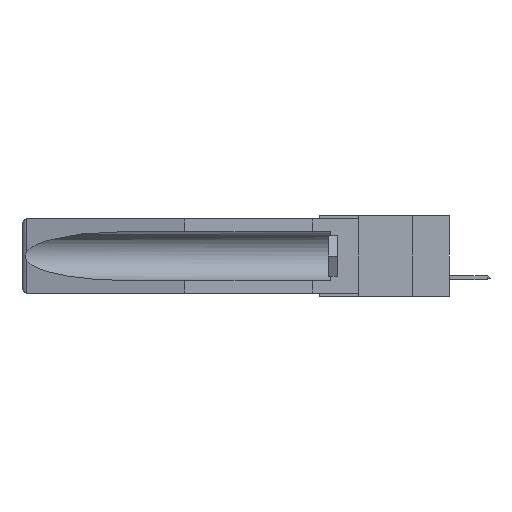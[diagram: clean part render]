
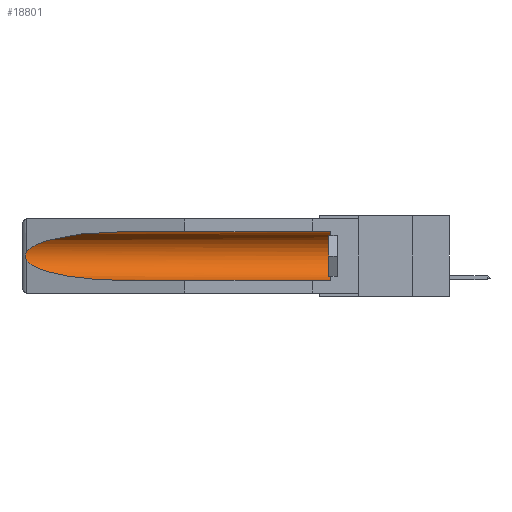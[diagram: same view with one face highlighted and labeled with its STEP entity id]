
A CAD part, left-side view. The second image highlights one B-rep face of the part: STEP entity #18801.
In plain terms, the highlighted cylindrical face has radius 2.857 mm (diameter 5.715 mm), a partial arc.
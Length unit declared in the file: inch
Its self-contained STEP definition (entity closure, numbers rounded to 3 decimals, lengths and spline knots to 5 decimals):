
#703 = VERTEX_POINT ( 'NONE', #5030 ) ;
#1342 = VERTEX_POINT ( 'NONE', #10967 ) ;
#1915 = EDGE_CURVE ( 'NONE', #703, #1342, #19641, .T. ) ;
#2113 = AXIS2_PLACEMENT_3D ( 'NONE', #3444, #9989, #6726 ) ;
#2271 = CIRCLE ( 'NONE', #9163, 0.1125 ) ;
#2732 = DIRECTION ( 'NONE',  ( 0., -1., 0. ) ) ;
#3019 = CARTESIAN_POINT ( 'NONE',  ( 0.25451, 1.48313, -0.09465 ) ) ;
#3235 = CARTESIAN_POINT ( 'NONE',  ( 0.155, 1.07973, -0.059 ) ) ;
#3444 = CARTESIAN_POINT ( 'NONE',  ( 0.155, -0.30754, -0.1715 ) ) ;
#3537 = ORIENTED_EDGE ( 'NONE', *, *, #13903, .F. ) ;
#4358 = LINE ( 'NONE', #16368, #6198 ) ;
#5024 = CARTESIAN_POINT ( 'NONE',  ( 0.26537, 1.52718, -0.14972 ) ) ;
#5030 = CARTESIAN_POINT ( 'NONE',  ( 0.155, 0.126, -0.059 ) ) ;
#6051 = CARTESIAN_POINT ( 'NONE',  ( 0.26654, 1.53092, -0.15636 ) ) ;
#6198 = VECTOR ( 'NONE', #9818, 39.37008 ) ;
#6726 = DIRECTION ( 'NONE',  ( 0., 0., 1. ) ) ;
#7001 = ORIENTED_EDGE ( 'NONE', *, *, #16975, .T. ) ;
#7324 = VERTEX_POINT ( 'NONE', #19945 ) ;
#7453 = CARTESIAN_POINT ( 'NONE',  ( 0.26537, 1.52718, -0.14972 ) ) ;
#7702 = CARTESIAN_POINT ( 'NONE',  ( 0.155, -0.30754, -0.059 ) ) ;
#7738 = CARTESIAN_POINT ( 'NONE',  ( 0.2675, 1.53308, -0.16763 ) ) ;
#7820 = EDGE_LOOP ( 'NONE', ( #7001, #20373, #15381, #3537, #12249, #8042 ) ) ;
#8042 = ORIENTED_EDGE ( 'NONE', *, *, #1915, .T. ) ;
#8125 = VECTOR ( 'NONE', #21120, 39.37008 ) ;
#8310 = CARTESIAN_POINT ( 'NONE',  ( 0.26537, 1.52718, -0.19328 ) ) ;
#9163 = AXIS2_PLACEMENT_3D ( 'NONE', #12665, #2732, #19387 ) ;
#9818 = DIRECTION ( 'NONE',  ( 0., 1., 0. ) ) ;
#9899 = FACE_OUTER_BOUND ( 'NONE', #7820, .T. ) ;
#9965 = B_SPLINE_CURVE_WITH_KNOTS ( 'NONE', 3,
 ( #7453, #12628, #6051, #15957, #7738, #17650, #15746, #10979, #19418, #17429 ),
 .UNSPECIFIED., .F., .F.,
 ( 4, 2, 2, 2, 4 ),
 ( 0., 0.00029, 0.00058, 0.00087, 0.00117 ),
 .UNSPECIFIED. ) ;
#9989 = DIRECTION ( 'NONE',  ( 0., 1., 0. ) ) ;
#10862 = VERTEX_POINT ( 'NONE', #20792 ) ;
#10967 = CARTESIAN_POINT ( 'NONE',  ( 0.155, 1.07973, -0.059 ) ) ;
#10979 = CARTESIAN_POINT ( 'NONE',  ( 0.26655, 1.53094, -0.18657 ) ) ;
#12249 = ORIENTED_EDGE ( 'NONE', *, *, #14209, .T. ) ;
#12628 = CARTESIAN_POINT ( 'NONE',  ( 0.26597, 1.52961, -0.15275 ) ) ;
#12665 = CARTESIAN_POINT ( 'NONE',  ( 0.155, 0.126, -0.1715 ) ) ;
#13320 = CARTESIAN_POINT ( 'NONE',  ( 0.26537, 1.52718, -0.19328 ) ) ;
#13903 = EDGE_CURVE ( 'NONE', #7324, #10862, #4358, .T. ) ;
#14111 = CYLINDRICAL_SURFACE ( 'NONE', #2113, 0.1125 ) ;
#14209 = EDGE_CURVE ( 'NONE', #7324, #703, #2271, .T. ) ;
#15381 = ORIENTED_EDGE ( 'NONE', *, *, #19057, .T. ) ;
#15453 =( BOUNDED_CURVE ( )  B_SPLINE_CURVE ( 3, ( #8310, #16805, #17589, #17446 ),
 .UNSPECIFIED., .F., .T. ) 
 B_SPLINE_CURVE_WITH_KNOTS ( ( 4, 4 ),
 ( 0.1948, 1.5708 ),
 .UNSPECIFIED. ) 
 CURVE ( )  GEOMETRIC_REPRESENTATION_ITEM ( )  RATIONAL_B_SPLINE_CURVE ( ( 1., 0.848, 0.848, 1. ) ) 
 REPRESENTATION_ITEM ( '' )  );
#15746 = CARTESIAN_POINT ( 'NONE',  ( 0.2673, 1.53269, -0.17917 ) ) ;
#15957 = CARTESIAN_POINT ( 'NONE',  ( 0.2673, 1.5327, -0.16383 ) ) ;
#16200 = VERTEX_POINT ( 'NONE', #13320 ) ;
#16368 = CARTESIAN_POINT ( 'NONE',  ( 0.155, -0.30754, -0.284 ) ) ;
#16494 = CARTESIAN_POINT ( 'NONE',  ( 0.26537, 1.52718, -0.14972 ) ) ;
#16805 = CARTESIAN_POINT ( 'NONE',  ( 0.25451, 1.48313, -0.24835 ) ) ;
#16975 = EDGE_CURVE ( 'NONE', #1342, #19453, #17045, .T. ) ;
#17045 =( BOUNDED_CURVE ( )  B_SPLINE_CURVE ( 3, ( #3235, #21423, #3019, #16494 ),
 .UNSPECIFIED., .F., .F. ) 
 B_SPLINE_CURVE_WITH_KNOTS ( ( 4, 4 ),
 ( 4.71239, 6.08839 ),
 .UNSPECIFIED. ) 
 CURVE ( )  GEOMETRIC_REPRESENTATION_ITEM ( )  RATIONAL_B_SPLINE_CURVE ( ( 1., 0.848, 0.848, 1. ) ) 
 REPRESENTATION_ITEM ( '' )  );
#17429 = CARTESIAN_POINT ( 'NONE',  ( 0.26537, 1.52718, -0.19328 ) ) ;
#17446 = CARTESIAN_POINT ( 'NONE',  ( 0.155, 1.07973, -0.284 ) ) ;
#17589 = CARTESIAN_POINT ( 'NONE',  ( 0.21114, 1.30732, -0.284 ) ) ;
#17650 = CARTESIAN_POINT ( 'NONE',  ( 0.2675, 1.53308, -0.17534 ) ) ;
#18801 = ADVANCED_FACE ( 'NONE', ( #9899 ), #14111, .F. ) ;
#19057 = EDGE_CURVE ( 'NONE', #16200, #10862, #15453, .T. ) ;
#19190 = EDGE_CURVE ( 'NONE', #19453, #16200, #9965, .T. ) ;
#19387 = DIRECTION ( 'NONE',  ( 0., 0., 1. ) ) ;
#19418 = CARTESIAN_POINT ( 'NONE',  ( 0.26597, 1.5296, -0.19026 ) ) ;
#19453 = VERTEX_POINT ( 'NONE', #5024 ) ;
#19641 = LINE ( 'NONE', #7702, #8125 ) ;
#19945 = CARTESIAN_POINT ( 'NONE',  ( 0.155, 0.126, -0.284 ) ) ;
#20373 = ORIENTED_EDGE ( 'NONE', *, *, #19190, .T. ) ;
#20792 = CARTESIAN_POINT ( 'NONE',  ( 0.155, 1.07973, -0.284 ) ) ;
#21120 = DIRECTION ( 'NONE',  ( 0., 1., 0. ) ) ;
#21423 = CARTESIAN_POINT ( 'NONE',  ( 0.21114, 1.30732, -0.059 ) ) ;
